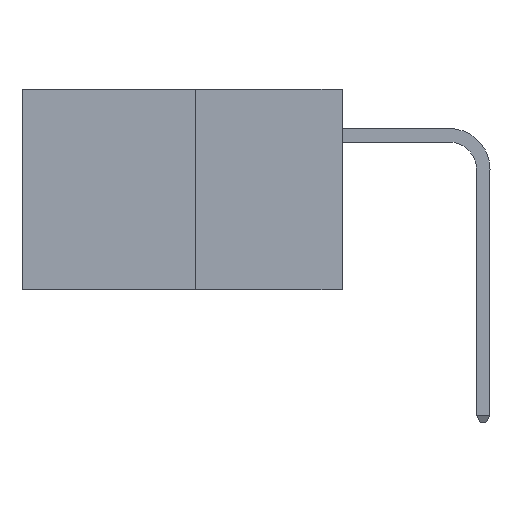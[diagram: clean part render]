
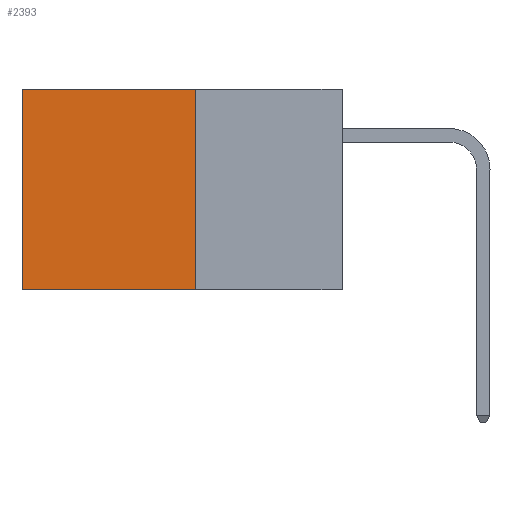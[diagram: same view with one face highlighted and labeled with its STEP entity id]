
A CAD part, left-side view. The second image highlights one B-rep face of the part: STEP entity #2393.
In plain terms, the highlighted planar face has unit normal (-1, 0, 0).
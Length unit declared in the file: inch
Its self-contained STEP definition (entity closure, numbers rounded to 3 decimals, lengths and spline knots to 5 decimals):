
#115 = CARTESIAN_POINT ( 'NONE',  ( 0.277, 0.27, -0.37 ) ) ;
#117 = EDGE_CURVE ( 'NONE', #1114, #2458, #7363, .T. ) ;
#377 = CARTESIAN_POINT ( 'NONE',  ( 0.277, 0.59, -0.37 ) ) ;
#707 = CARTESIAN_POINT ( 'NONE',  ( 0.277, 0.27, 0. ) ) ;
#1114 = VERTEX_POINT ( 'NONE', #10315 ) ;
#1369 = CARTESIAN_POINT ( 'NONE',  ( 0.277, 0.27, -0.37 ) ) ;
#1374 = DIRECTION ( 'NONE',  ( 0., 0., -1. ) ) ;
#1682 = DIRECTION ( 'NONE',  ( 0., 1., 0. ) ) ;
#2133 = VECTOR ( 'NONE', #8570, 39.37008 ) ;
#2393 = ADVANCED_FACE ( 'NONE', ( #10096 ), #3511, .F. ) ;
#2458 = VERTEX_POINT ( 'NONE', #2773 ) ;
#2529 = VERTEX_POINT ( 'NONE', #6528 ) ;
#2752 = ORIENTED_EDGE ( 'NONE', *, *, #4620, .T. ) ;
#2773 = CARTESIAN_POINT ( 'NONE',  ( 0.277, 0.27, -0.37 ) ) ;
#3240 = EDGE_CURVE ( 'NONE', #2458, #6937, #4277, .T. ) ;
#3342 = DIRECTION ( 'NONE',  ( 0., 0., -1. ) ) ;
#3511 = PLANE ( 'NONE',  #4934 ) ;
#4277 = LINE ( 'NONE', #115, #10515 ) ;
#4325 = EDGE_CURVE ( 'NONE', #1114, #2529, #7427, .T. ) ;
#4439 = DIRECTION ( 'NONE',  ( 1., 0., 0. ) ) ;
#4475 = EDGE_LOOP ( 'NONE', ( #2752, #7776, #7722, #7540 ) ) ;
#4620 = EDGE_CURVE ( 'NONE', #2529, #6937, #4998, .T. ) ;
#4934 = AXIS2_PLACEMENT_3D ( 'NONE', #9104, #4439, #3342 ) ;
#4998 = LINE ( 'NONE', #377, #9282 ) ;
#5015 = VECTOR ( 'NONE', #1682, 39.37008 ) ;
#5211 = CARTESIAN_POINT ( 'NONE',  ( 0.277, 0.59, -0.37 ) ) ;
#6528 = CARTESIAN_POINT ( 'NONE',  ( 0.277, 0.59, 0. ) ) ;
#6937 = VERTEX_POINT ( 'NONE', #5211 ) ;
#7363 = LINE ( 'NONE', #1369, #2133 ) ;
#7427 = LINE ( 'NONE', #707, #5015 ) ;
#7540 = ORIENTED_EDGE ( 'NONE', *, *, #4325, .T. ) ;
#7722 = ORIENTED_EDGE ( 'NONE', *, *, #117, .F. ) ;
#7776 = ORIENTED_EDGE ( 'NONE', *, *, #3240, .F. ) ;
#7964 = DIRECTION ( 'NONE',  ( 0., 1., 0. ) ) ;
#8570 = DIRECTION ( 'NONE',  ( 0., 0., -1. ) ) ;
#9104 = CARTESIAN_POINT ( 'NONE',  ( 0.277, 0.27, -0.37 ) ) ;
#9282 = VECTOR ( 'NONE', #1374, 39.37008 ) ;
#10096 = FACE_OUTER_BOUND ( 'NONE', #4475, .T. ) ;
#10315 = CARTESIAN_POINT ( 'NONE',  ( 0.277, 0.27, 0. ) ) ;
#10515 = VECTOR ( 'NONE', #7964, 39.37008 ) ;
